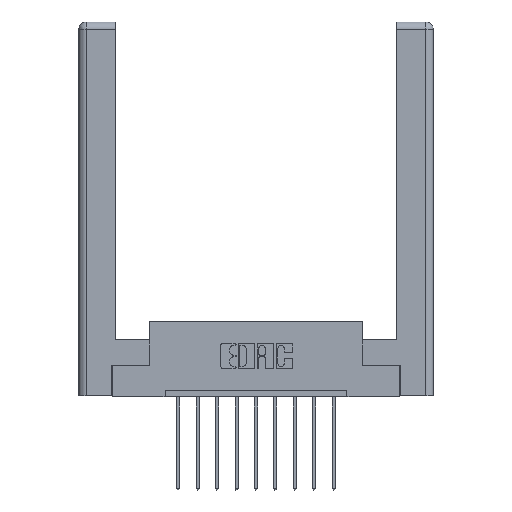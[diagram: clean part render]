
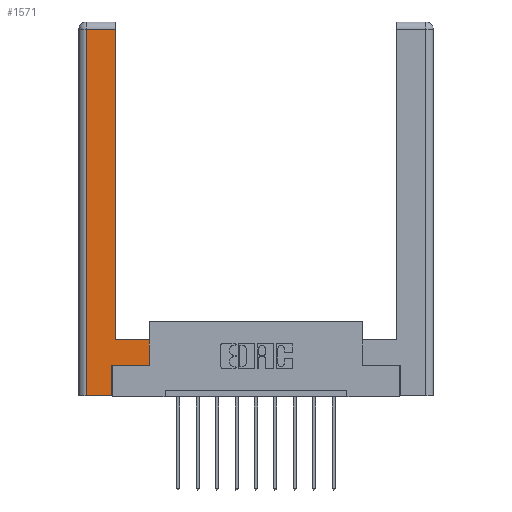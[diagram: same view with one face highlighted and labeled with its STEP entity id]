
A CAD part, top view. The second image highlights one B-rep face of the part: STEP entity #1571.
In plain terms, the highlighted planar face has unit normal (0, 0, 1).
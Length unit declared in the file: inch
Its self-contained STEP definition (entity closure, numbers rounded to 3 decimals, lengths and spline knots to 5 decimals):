
#280 = VECTOR ( 'NONE', #1397, 39.37008 ) ;
#789 = VERTEX_POINT ( 'NONE', #6529 ) ;
#875 = DIRECTION ( 'NONE',  ( 0., -1., 0. ) ) ;
#933 = VERTEX_POINT ( 'NONE', #13332 ) ;
#1092 = CARTESIAN_POINT ( 'NONE',  ( 0.0615, 2.94, 0. ) ) ;
#1100 = ORIENTED_EDGE ( 'NONE', *, *, #7454, .T. ) ;
#1125 = LINE ( 'NONE', #13529, #12505 ) ;
#1136 = DIRECTION ( 'NONE',  ( -1., 0., 0. ) ) ;
#1308 = VECTOR ( 'NONE', #1416, 39.37008 ) ;
#1329 = FACE_OUTER_BOUND ( 'NONE', #4581, .T. ) ;
#1376 = VECTOR ( 'NONE', #1136, 39.37008 ) ;
#1397 = DIRECTION ( 'NONE',  ( 1., 0., 0. ) ) ;
#1416 = DIRECTION ( 'NONE',  ( -1., 0., 0. ) ) ;
#1446 = AXIS2_PLACEMENT_3D ( 'NONE', #9411, #10442, #8416 ) ;
#1484 = EDGE_CURVE ( 'NONE', #11098, #8421, #5132, .T. ) ;
#1571 = ADVANCED_FACE ( 'NONE', ( #1329 ), #11469, .F. ) ;
#2310 = ORIENTED_EDGE ( 'NONE', *, *, #2784, .T. ) ;
#2595 = CARTESIAN_POINT ( 'NONE',  ( 0.565, 0.45, 0. ) ) ;
#2784 = EDGE_CURVE ( 'NONE', #2792, #9533, #4102, .T. ) ;
#2792 = VERTEX_POINT ( 'NONE', #2595 ) ;
#3664 = CARTESIAN_POINT ( 'NONE',  ( 0.565, 0.245, 0. ) ) ;
#4102 = LINE ( 'NONE', #7741, #1308 ) ;
#4359 = EDGE_CURVE ( 'NONE', #789, #11098, #7195, .T. ) ;
#4389 = VERTEX_POINT ( 'NONE', #13440 ) ;
#4426 = LINE ( 'NONE', #13481, #13512 ) ;
#4581 = EDGE_LOOP ( 'NONE', ( #6262, #6963, #8383, #11528, #10870, #1100, #7405, #2310 ) ) ;
#5132 = LINE ( 'NONE', #12697, #13232 ) ;
#5638 = VERTEX_POINT ( 'NONE', #3664 ) ;
#6226 = DIRECTION ( 'NONE',  ( 0., 1., 0. ) ) ;
#6262 = ORIENTED_EDGE ( 'NONE', *, *, #10137, .T. ) ;
#6489 = EDGE_CURVE ( 'NONE', #5638, #2792, #7629, .T. ) ;
#6529 = CARTESIAN_POINT ( 'NONE',  ( 0.0615, 0., 0. ) ) ;
#6963 = ORIENTED_EDGE ( 'NONE', *, *, #12431, .T. ) ;
#7036 = LINE ( 'NONE', #8167, #280 ) ;
#7195 = LINE ( 'NONE', #10318, #12484 ) ;
#7405 = ORIENTED_EDGE ( 'NONE', *, *, #6489, .T. ) ;
#7454 = EDGE_CURVE ( 'NONE', #8421, #5638, #7036, .T. ) ;
#7629 = LINE ( 'NONE', #9818, #13248 ) ;
#7741 = CARTESIAN_POINT ( 'NONE',  ( 0.295, 0.45, 0. ) ) ;
#8167 = CARTESIAN_POINT ( 'NONE',  ( 0.565, 0.245, 0. ) ) ;
#8383 = ORIENTED_EDGE ( 'NONE', *, *, #9039, .T. ) ;
#8416 = DIRECTION ( 'NONE',  ( -1., 0., 0. ) ) ;
#8421 = VERTEX_POINT ( 'NONE', #13606 ) ;
#8526 = DIRECTION ( 'NONE',  ( 0., 1., 0. ) ) ;
#9039 = EDGE_CURVE ( 'NONE', #4389, #789, #4426, .T. ) ;
#9047 = DIRECTION ( 'NONE',  ( 0., 1., 0. ) ) ;
#9411 = CARTESIAN_POINT ( 'NONE',  ( 0., 0., 0. ) ) ;
#9499 = LINE ( 'NONE', #1092, #1376 ) ;
#9533 = VERTEX_POINT ( 'NONE', #13124 ) ;
#9818 = CARTESIAN_POINT ( 'NONE',  ( 0.565, 0.45, 0. ) ) ;
#10137 = EDGE_CURVE ( 'NONE', #9533, #933, #1125, .T. ) ;
#10318 = CARTESIAN_POINT ( 'NONE',  ( 0.265, 0., 0. ) ) ;
#10442 = DIRECTION ( 'NONE',  ( 0., 0., -1. ) ) ;
#10870 = ORIENTED_EDGE ( 'NONE', *, *, #1484, .T. ) ;
#11098 = VERTEX_POINT ( 'NONE', #12936 ) ;
#11469 = PLANE ( 'NONE',  #1446 ) ;
#11528 = ORIENTED_EDGE ( 'NONE', *, *, #4359, .T. ) ;
#12431 = EDGE_CURVE ( 'NONE', #933, #4389, #9499, .T. ) ;
#12484 = VECTOR ( 'NONE', #13531, 39.37008 ) ;
#12505 = VECTOR ( 'NONE', #9047, 39.37008 ) ;
#12697 = CARTESIAN_POINT ( 'NONE',  ( 0.265, 0.245, 0. ) ) ;
#12936 = CARTESIAN_POINT ( 'NONE',  ( 0.265, 0., 0. ) ) ;
#13124 = CARTESIAN_POINT ( 'NONE',  ( 0.295, 0.45, 0. ) ) ;
#13232 = VECTOR ( 'NONE', #8526, 39.37008 ) ;
#13248 = VECTOR ( 'NONE', #6226, 39.37008 ) ;
#13332 = CARTESIAN_POINT ( 'NONE',  ( 0.295, 2.94, 0. ) ) ;
#13440 = CARTESIAN_POINT ( 'NONE',  ( 0.0615, 2.94, 0. ) ) ;
#13481 = CARTESIAN_POINT ( 'NONE',  ( 0.0615, 0., 0. ) ) ;
#13512 = VECTOR ( 'NONE', #875, 39.37008 ) ;
#13529 = CARTESIAN_POINT ( 'NONE',  ( 0.295, 3., 0. ) ) ;
#13531 = DIRECTION ( 'NONE',  ( 1., 0., 0. ) ) ;
#13606 = CARTESIAN_POINT ( 'NONE',  ( 0.265, 0.245, 0. ) ) ;
